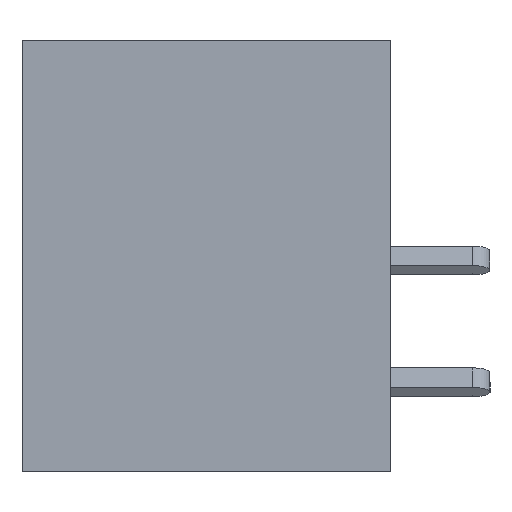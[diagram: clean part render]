
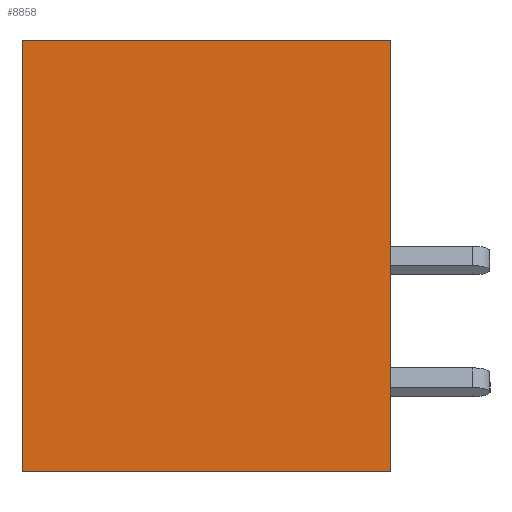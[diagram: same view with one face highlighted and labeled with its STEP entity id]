
A CAD part, left-side view. The second image highlights one B-rep face of the part: STEP entity #8858.
In plain terms, the highlighted planar face has unit normal (-1, 0, 0).
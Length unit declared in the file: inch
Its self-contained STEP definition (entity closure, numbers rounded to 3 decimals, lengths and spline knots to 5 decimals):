
#344 = VECTOR ( 'NONE', #7831, 39.37008 ) ;
#696 = CARTESIAN_POINT ( 'NONE',  ( 0., 0.453, 0. ) ) ;
#1014 = VERTEX_POINT ( 'NONE', #12693 ) ;
#1864 = LINE ( 'NONE', #4858, #2271 ) ;
#2271 = VECTOR ( 'NONE', #15284, 39.37008 ) ;
#2373 = ORIENTED_EDGE ( 'NONE', *, *, #14328, .F. ) ;
#3026 = LINE ( 'NONE', #11909, #344 ) ;
#3241 = CARTESIAN_POINT ( 'NONE',  ( 0., 0., 0. ) ) ;
#3539 = DIRECTION ( 'NONE',  ( 0., 0., -1. ) ) ;
#3557 = EDGE_CURVE ( 'NONE', #16424, #15886, #5952, .T. ) ;
#4858 = CARTESIAN_POINT ( 'NONE',  ( 0., 0.453, 0. ) ) ;
#5019 = CARTESIAN_POINT ( 'NONE',  ( 0., 0.453, 0. ) ) ;
#5081 = ORIENTED_EDGE ( 'NONE', *, *, #15815, .F. ) ;
#5094 = VECTOR ( 'NONE', #8400, 39.37008 ) ;
#5186 = AXIS2_PLACEMENT_3D ( 'NONE', #5019, #10281, #3539 ) ;
#5698 = VERTEX_POINT ( 'NONE', #696 ) ;
#5952 = LINE ( 'NONE', #11306, #15767 ) ;
#7831 = DIRECTION ( 'NONE',  ( 0., -1., 0. ) ) ;
#8400 = DIRECTION ( 'NONE',  ( 0., 0., 1. ) ) ;
#8588 = LINE ( 'NONE', #3241, #5094 ) ;
#8858 = ADVANCED_FACE ( 'NONE', ( #9353 ), #9328, .F. ) ;
#9328 = PLANE ( 'NONE',  #5186 ) ;
#9353 = FACE_OUTER_BOUND ( 'NONE', #11532, .T. ) ;
#10033 = DIRECTION ( 'NONE',  ( 0., -1., 0. ) ) ;
#10281 = DIRECTION ( 'NONE',  ( 1., 0., 0. ) ) ;
#10627 = ORIENTED_EDGE ( 'NONE', *, *, #3557, .T. ) ;
#11306 = CARTESIAN_POINT ( 'NONE',  ( 0., 0.453, -0.531 ) ) ;
#11532 = EDGE_LOOP ( 'NONE', ( #13959, #5081, #2373, #10627 ) ) ;
#11909 = CARTESIAN_POINT ( 'NONE',  ( 0., 0.453, 0. ) ) ;
#12693 = CARTESIAN_POINT ( 'NONE',  ( 0., 0., 0. ) ) ;
#12977 = CARTESIAN_POINT ( 'NONE',  ( 0., 0.453, -0.531 ) ) ;
#13959 = ORIENTED_EDGE ( 'NONE', *, *, #16119, .T. ) ;
#14328 = EDGE_CURVE ( 'NONE', #16424, #5698, #1864, .T. ) ;
#14629 = CARTESIAN_POINT ( 'NONE',  ( 0., 0., -0.531 ) ) ;
#15284 = DIRECTION ( 'NONE',  ( 0., 0., 1. ) ) ;
#15767 = VECTOR ( 'NONE', #10033, 39.37008 ) ;
#15815 = EDGE_CURVE ( 'NONE', #5698, #1014, #3026, .T. ) ;
#15886 = VERTEX_POINT ( 'NONE', #14629 ) ;
#16119 = EDGE_CURVE ( 'NONE', #15886, #1014, #8588, .T. ) ;
#16424 = VERTEX_POINT ( 'NONE', #12977 ) ;
